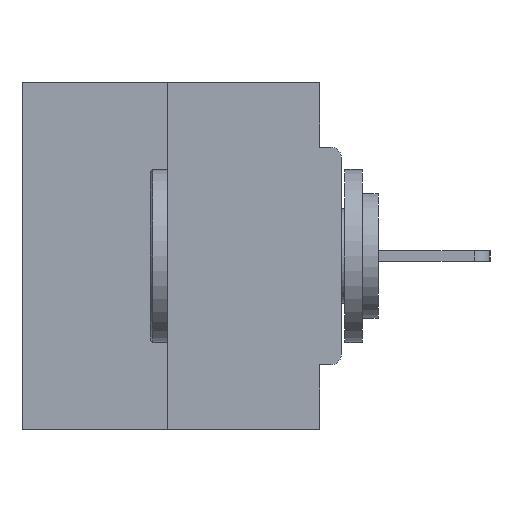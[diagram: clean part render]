
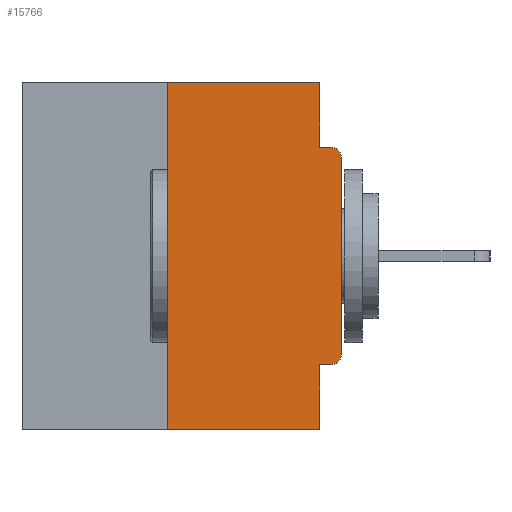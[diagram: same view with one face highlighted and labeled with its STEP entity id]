
A CAD part, left-side view. The second image highlights one B-rep face of the part: STEP entity #15766.
In plain terms, the highlighted planar face has unit normal (-1, 0, 0).
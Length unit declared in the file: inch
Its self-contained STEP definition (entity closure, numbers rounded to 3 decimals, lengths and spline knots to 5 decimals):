
#139 = VECTOR ( 'NONE', #19596, 39.37008 ) ;
#219 = LINE ( 'NONE', #21314, #23552 ) ;
#315 = EDGE_CURVE ( 'NONE', #2107, #2619, #219, .T. ) ;
#914 = CARTESIAN_POINT ( 'NONE',  ( 0., 0.46, 0. ) ) ;
#1356 = CARTESIAN_POINT ( 'NONE',  ( 0., 0.25, 0. ) ) ;
#1421 = VECTOR ( 'NONE', #16502, 39.37008 ) ;
#2107 = VERTEX_POINT ( 'NONE', #29871 ) ;
#2619 = VERTEX_POINT ( 'NONE', #4687 ) ;
#3116 = ORIENTED_EDGE ( 'NONE', *, *, #4235, .F. ) ;
#4235 = EDGE_CURVE ( 'NONE', #23727, #32053, #9700, .T. ) ;
#4529 = CIRCLE ( 'NONE', #14344, 0.015 ) ;
#4566 = CARTESIAN_POINT ( 'NONE',  ( 0., 0.46, 0. ) ) ;
#4687 = CARTESIAN_POINT ( 'NONE',  ( 0., 0., -0.1085 ) ) ;
#5489 = CARTESIAN_POINT ( 'NONE',  ( 0., 0.015, -0.0935 ) ) ;
#5926 = LINE ( 'NONE', #19121, #21788 ) ;
#6417 = CIRCLE ( 'NONE', #34133, 0.015 ) ;
#6714 = VERTEX_POINT ( 'NONE', #19275 ) ;
#7102 = CARTESIAN_POINT ( 'NONE',  ( 0., 0.031, -0.5 ) ) ;
#7415 = VERTEX_POINT ( 'NONE', #5489 ) ;
#7535 = CARTESIAN_POINT ( 'NONE',  ( 0., 0.25, -0.5 ) ) ;
#7916 = VERTEX_POINT ( 'NONE', #7535 ) ;
#9700 = LINE ( 'NONE', #18548, #23771 ) ;
#9958 = ORIENTED_EDGE ( 'NONE', *, *, #315, .T. ) ;
#10577 = DIRECTION ( 'NONE',  ( -1., 0., 0. ) ) ;
#10680 = ORIENTED_EDGE ( 'NONE', *, *, #29930, .F. ) ;
#11878 = EDGE_CURVE ( 'NONE', #6714, #2107, #6417, .T. ) ;
#11972 = ORIENTED_EDGE ( 'NONE', *, *, #23166, .F. ) ;
#13276 = DIRECTION ( 'NONE',  ( 0., 0., 1. ) ) ;
#13700 = EDGE_CURVE ( 'NONE', #14446, #16318, #13797, .T. ) ;
#13797 = LINE ( 'NONE', #16271, #35074 ) ;
#14344 = AXIS2_PLACEMENT_3D ( 'NONE', #14852, #34262, #17678 ) ;
#14446 = VERTEX_POINT ( 'NONE', #21175 ) ;
#14852 = CARTESIAN_POINT ( 'NONE',  ( 0., 0.015, -0.1085 ) ) ;
#15180 = ORIENTED_EDGE ( 'NONE', *, *, #13700, .F. ) ;
#15717 = ORIENTED_EDGE ( 'NONE', *, *, #17454, .T. ) ;
#15766 = ADVANCED_FACE ( 'NONE', ( #34203 ), #29797, .F. ) ;
#15922 = DIRECTION ( 'NONE',  ( 0., 0., -1. ) ) ;
#16271 = CARTESIAN_POINT ( 'NONE',  ( 0., 0.031, -0.5 ) ) ;
#16299 = VECTOR ( 'NONE', #25835, 39.37008 ) ;
#16318 = VERTEX_POINT ( 'NONE', #7102 ) ;
#16502 = DIRECTION ( 'NONE',  ( 0., 0., 1. ) ) ;
#17248 = CARTESIAN_POINT ( 'NONE',  ( 0., 0.031, -0.0935 ) ) ;
#17265 = ORIENTED_EDGE ( 'NONE', *, *, #30520, .F. ) ;
#17454 = EDGE_CURVE ( 'NONE', #7916, #16318, #30229, .T. ) ;
#17565 = CARTESIAN_POINT ( 'NONE',  ( 0., 0.46, -0.5 ) ) ;
#17678 = DIRECTION ( 'NONE',  ( 0., 0., -1. ) ) ;
#17814 = DIRECTION ( 'NONE',  ( 0., 0., -1. ) ) ;
#18548 = CARTESIAN_POINT ( 'NONE',  ( 0., 0.031, 0. ) ) ;
#19121 = CARTESIAN_POINT ( 'NONE',  ( 0., 0., -0.0935 ) ) ;
#19275 = CARTESIAN_POINT ( 'NONE',  ( 0., 0.015, -0.4065 ) ) ;
#19339 = EDGE_CURVE ( 'NONE', #20589, #23727, #32718, .T. ) ;
#19596 = DIRECTION ( 'NONE',  ( 0., 1., 0. ) ) ;
#19820 = EDGE_LOOP ( 'NONE', ( #22644, #17265, #15717, #15180, #10680, #27993, #9958, #25395, #11972, #3116 ) ) ;
#20589 = VERTEX_POINT ( 'NONE', #1356 ) ;
#20633 = DIRECTION ( 'NONE',  ( 0., -1., 0. ) ) ;
#21175 = CARTESIAN_POINT ( 'NONE',  ( 0., 0.031, -0.4065 ) ) ;
#21314 = CARTESIAN_POINT ( 'NONE',  ( 0., 0., 0. ) ) ;
#21788 = VECTOR ( 'NONE', #24698, 39.37008 ) ;
#22284 = CARTESIAN_POINT ( 'NONE',  ( 0., 0., -0.4065 ) ) ;
#22644 = ORIENTED_EDGE ( 'NONE', *, *, #19339, .F. ) ;
#23166 = EDGE_CURVE ( 'NONE', #32053, #7415, #5926, .T. ) ;
#23552 = VECTOR ( 'NONE', #13276, 39.37008 ) ;
#23727 = VERTEX_POINT ( 'NONE', #30391 ) ;
#23771 = VECTOR ( 'NONE', #17814, 39.37008 ) ;
#23860 = LINE ( 'NONE', #27574, #1421 ) ;
#24698 = DIRECTION ( 'NONE',  ( 0., -1., 0. ) ) ;
#25350 = VECTOR ( 'NONE', #20633, 39.37008 ) ;
#25395 = ORIENTED_EDGE ( 'NONE', *, *, #31294, .T. ) ;
#25835 = DIRECTION ( 'NONE',  ( 0., -1., 0. ) ) ;
#27332 = CARTESIAN_POINT ( 'NONE',  ( 0., 0.015, -0.3915 ) ) ;
#27574 = CARTESIAN_POINT ( 'NONE',  ( 0., 0.25, 0. ) ) ;
#27993 = ORIENTED_EDGE ( 'NONE', *, *, #11878, .T. ) ;
#29797 = PLANE ( 'NONE',  #30109 ) ;
#29871 = CARTESIAN_POINT ( 'NONE',  ( 0., 0., -0.3915 ) ) ;
#29930 = EDGE_CURVE ( 'NONE', #6714, #14446, #30000, .T. ) ;
#30000 = LINE ( 'NONE', #22284, #139 ) ;
#30109 = AXIS2_PLACEMENT_3D ( 'NONE', #4566, #32569, #15922 ) ;
#30133 = DIRECTION ( 'NONE',  ( 0., 0., -1. ) ) ;
#30229 = LINE ( 'NONE', #17565, #16299 ) ;
#30391 = CARTESIAN_POINT ( 'NONE',  ( 0., 0.031, 0. ) ) ;
#30520 = EDGE_CURVE ( 'NONE', #7916, #20589, #23860, .T. ) ;
#31294 = EDGE_CURVE ( 'NONE', #2619, #7415, #4529, .T. ) ;
#32053 = VERTEX_POINT ( 'NONE', #17248 ) ;
#32569 = DIRECTION ( 'NONE',  ( 1., 0., 0. ) ) ;
#32718 = LINE ( 'NONE', #914, #25350 ) ;
#34133 = AXIS2_PLACEMENT_3D ( 'NONE', #27332, #10577, #30133 ) ;
#34203 = FACE_OUTER_BOUND ( 'NONE', #19820, .T. ) ;
#34262 = DIRECTION ( 'NONE',  ( -1., 0., 0. ) ) ;
#35074 = VECTOR ( 'NONE', #35506, 39.37008 ) ;
#35506 = DIRECTION ( 'NONE',  ( 0., 0., -1. ) ) ;
